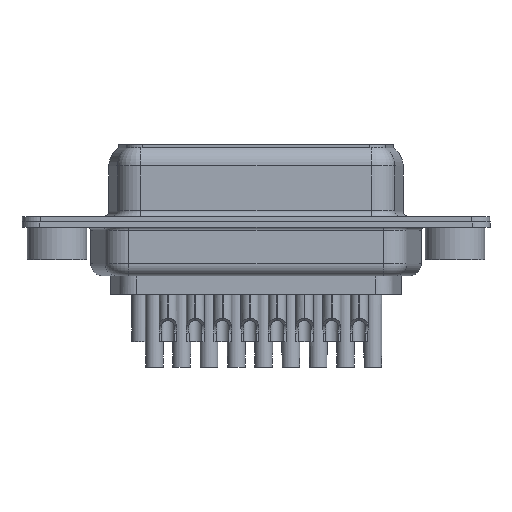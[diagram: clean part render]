
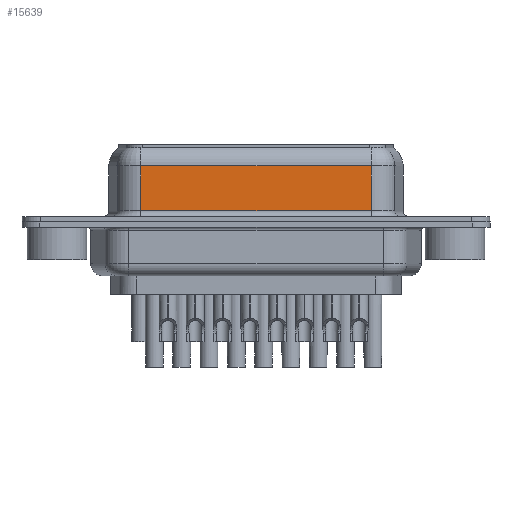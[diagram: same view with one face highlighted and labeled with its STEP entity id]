
A CAD part, front view. The second image highlights one B-rep face of the part: STEP entity #15639.
In plain terms, the highlighted planar face has unit normal (0, -1, 0).
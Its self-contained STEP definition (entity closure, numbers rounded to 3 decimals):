
#748 = DIRECTION ( 'NONE',  ( 0., 0., 1. ) ) ;
#1102 = ORIENTED_EDGE ( 'NONE', *, *, #16896, .T. ) ;
#1144 = CARTESIAN_POINT ( 'NONE',  ( 26.297, -3.95, 0.95 ) ) ;
#2348 = CARTESIAN_POINT ( 'NONE',  ( 7.023, -3.95, 4.7 ) ) ;
#3717 = VECTOR ( 'NONE', #4654, 1000. ) ;
#3900 = CARTESIAN_POINT ( 'NONE',  ( 26.297, -3.95, 6.45 ) ) ;
#4654 = DIRECTION ( 'NONE',  ( -1., 0., 0. ) ) ;
#5673 = DIRECTION ( 'NONE',  ( 0., 0., -1. ) ) ;
#6711 = EDGE_LOOP ( 'NONE', ( #8741, #12296, #16701, #1102 ) ) ;
#7507 = VECTOR ( 'NONE', #22064, 1000. ) ;
#8313 = LINE ( 'NONE', #3900, #9549 ) ;
#8741 = ORIENTED_EDGE ( 'NONE', *, *, #11423, .F. ) ;
#9549 = VECTOR ( 'NONE', #5673, 1000. ) ;
#10297 = LINE ( 'NONE', #23672, #7507 ) ;
#11423 = EDGE_CURVE ( 'NONE', #28055, #16877, #8313, .T. ) ;
#12296 = ORIENTED_EDGE ( 'NONE', *, *, #13211, .T. ) ;
#12747 = DIRECTION ( 'NONE',  ( 1., 0., 0. ) ) ;
#13211 = EDGE_CURVE ( 'NONE', #28055, #19560, #25185, .T. ) ;
#13949 = EDGE_CURVE ( 'NONE', #19560, #21215, #10297, .T. ) ;
#15639 = ADVANCED_FACE ( 'NONE', ( #20871 ), #23066, .F. ) ;
#16577 = LINE ( 'NONE', #1144, #20216 ) ;
#16701 = ORIENTED_EDGE ( 'NONE', *, *, #13949, .T. ) ;
#16877 = VERTEX_POINT ( 'NONE', #20543 ) ;
#16896 = EDGE_CURVE ( 'NONE', #21215, #16877, #16577, .T. ) ;
#18285 = CARTESIAN_POINT ( 'NONE',  ( 26.297, -3.95, 4.7 ) ) ;
#19560 = VERTEX_POINT ( 'NONE', #2348 ) ;
#19693 = AXIS2_PLACEMENT_3D ( 'NONE', #20721, #25406, #748 ) ;
#20216 = VECTOR ( 'NONE', #12747, 1000. ) ;
#20543 = CARTESIAN_POINT ( 'NONE',  ( 26.297, -3.95, 0.95 ) ) ;
#20721 = CARTESIAN_POINT ( 'NONE',  ( 26.297, -3.95, 6.45 ) ) ;
#20871 = FACE_OUTER_BOUND ( 'NONE', #6711, .T. ) ;
#21215 = VERTEX_POINT ( 'NONE', #26813 ) ;
#22064 = DIRECTION ( 'NONE',  ( 0., 0., -1. ) ) ;
#23066 = PLANE ( 'NONE',  #19693 ) ;
#23672 = CARTESIAN_POINT ( 'NONE',  ( 7.023, -3.95, 6.45 ) ) ;
#25185 = LINE ( 'NONE', #26979, #3717 ) ;
#25406 = DIRECTION ( 'NONE',  ( 0., 1., 0. ) ) ;
#26813 = CARTESIAN_POINT ( 'NONE',  ( 7.023, -3.95, 0.95 ) ) ;
#26979 = CARTESIAN_POINT ( 'NONE',  ( 26.297, -3.95, 4.7 ) ) ;
#28055 = VERTEX_POINT ( 'NONE', #18285 ) ;
